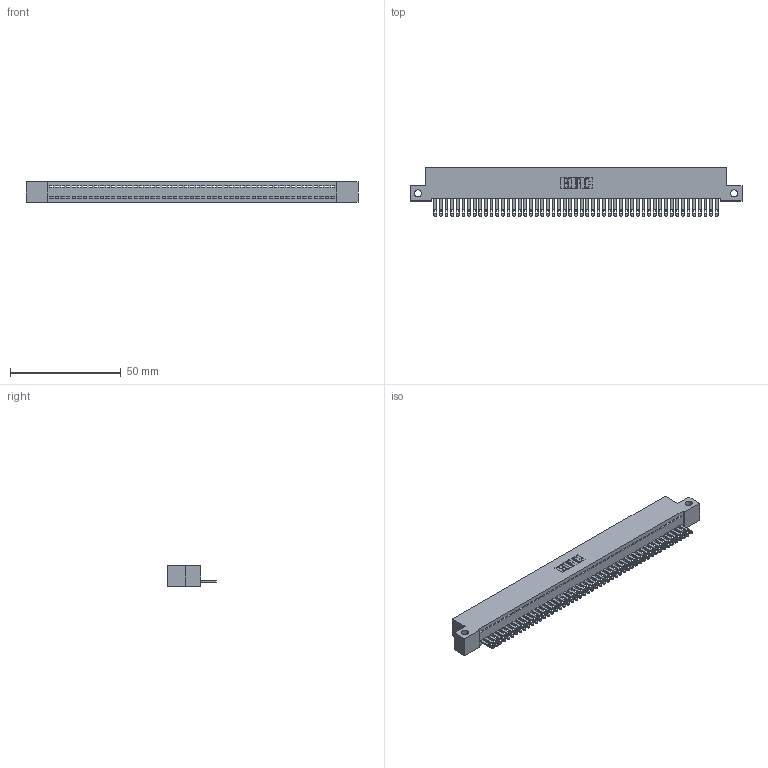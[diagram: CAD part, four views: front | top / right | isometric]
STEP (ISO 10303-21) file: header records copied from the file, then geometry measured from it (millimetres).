
FILE_DESCRIPTION (( 'STEP AP203' ), '1' );
FILE_NAME ('892-051-500-112.STEP', '2020-09-21T18:00:00', ( '' ), ( '' ), 'SwSTEP 2.0', 'SolidWorks 2020', '' );
FILE_SCHEMA (( 'CONFIG_CONTROL_DESIGN' ));
Length unit declared in the file: inch
Products named in the file (3): 842 Part_Side Mount; 892-051-500-112; 345-292-001_345-293-100
Assembly tree (52 placements, depth 2):
  892-051-500-112
    842 Part_Side Mount
    345-292-001_345-293-100  x51
Bounding box: 149.86 x 21.85 x 9.4 mm (x, y, z)
Volume: 13130.5 mm3; surface area: 19386.9 mm2
Topology: 52 solids, 52 shells, 2864 faces, 8867 edges, 5910 vertices
Faces by surface type: plane 1902, cylinder 962
Entity records: 29815 total; most frequent: CARTESIAN_POINT 5147, ORIENTED_EDGE 5134, DIRECTION 4325, EDGE_CURVE 2567, VECTOR 2435, LINE 2435, VERTEX_POINT 1710, AXIS2_PLACEMENT_3D 945
